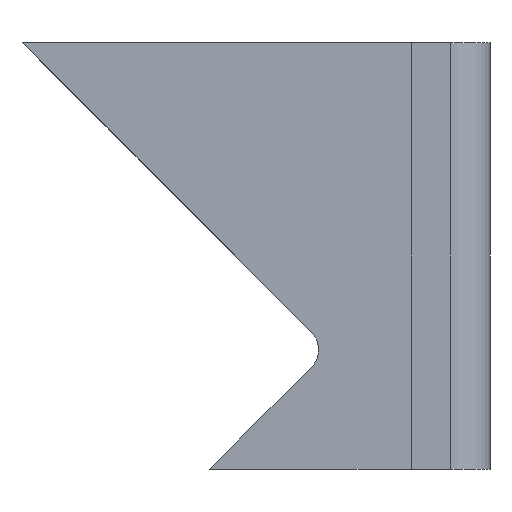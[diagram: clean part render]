
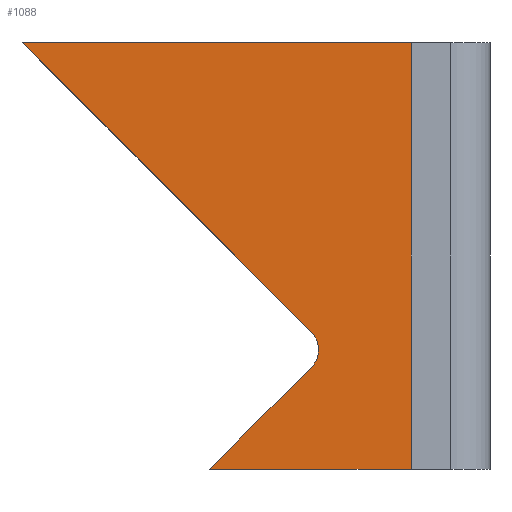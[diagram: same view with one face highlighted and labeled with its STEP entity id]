
A CAD part, front view. The second image highlights one B-rep face of the part: STEP entity #1088.
In plain terms, the highlighted planar face has unit normal (0, -1, 0).
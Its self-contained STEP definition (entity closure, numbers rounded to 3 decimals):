
#139 = VERTEX_POINT('',#140);
#140 = CARTESIAN_POINT('',(4.873,-25.4,-5.818));
#154 = PLANE('',#155);
#155 = AXIS2_PLACEMENT_3D('',#156,#157,#158);
#156 = CARTESIAN_POINT('',(-0.064,-25.4,-5.818));
#157 = DIRECTION('',(0.,0.,1.));
#158 = DIRECTION('',(-1.,0.,0.));
#181 = PLANE('',#182);
#182 = AXIS2_PLACEMENT_3D('',#183,#184,#185);
#183 = CARTESIAN_POINT('',(-5.84,-25.4,5.924));
#184 = DIRECTION('',(0.,-1.,0.));
#185 = DIRECTION('',(0.,0.,-1.));
#345 = CYLINDRICAL_SURFACE('',#346,0.635);
#346 = AXIS2_PLACEMENT_3D('',#347,#348,#349);
#347 = CARTESIAN_POINT('',(1.89,-25.4,-2.788));
#348 = DIRECTION('',(0.,-1.,0.));
#349 = DIRECTION('',(-1.,0.,0.));
#395 = PLANE('',#396);
#396 = AXIS2_PLACEMENT_3D('',#397,#398,#399);
#397 = CARTESIAN_POINT('',(-3.215,-25.4,-8.791));
#398 = DIRECTION('',(0.707,0.,-0.707));
#399 = DIRECTION('',(0.707,0.,0.707));
#445 = PLANE('',#446);
#446 = AXIS2_PLACEMENT_3D('',#447,#448,#449);
#447 = CARTESIAN_POINT('',(-0.064,-25.4,5.));
#448 = DIRECTION('',(0.,0.,-1.));
#449 = DIRECTION('',(1.,0.,0.));
#471 = PLANE('',#472);
#472 = AXIS2_PLACEMENT_3D('',#473,#474,#475);
#473 = CARTESIAN_POINT('',(5.939,-25.4,-5.939));
#474 = DIRECTION('',(-0.707,0.,-0.707));
#475 = DIRECTION('',(0.707,0.,-0.707));
#487 = VERTEX_POINT('',#488);
#488 = CARTESIAN_POINT('',(4.873,-25.4,5.));
#584 = VERTEX_POINT('',#585);
#585 = CARTESIAN_POINT('',(-0.242,-25.4,-5.818));
#606 = EDGE_CURVE('',#584,#139,#607,.T.);
#607 = SURFACE_CURVE('',#608,(#612,#619),.PCURVE_S1.);
#608 = LINE('',#609,#610);
#609 = CARTESIAN_POINT('',(-0.064,-25.4,-5.818));
#610 = VECTOR('',#611,1.);
#611 = DIRECTION('',(1.,0.,0.));
#612 = PCURVE('',#154,#613);
#613 = DEFINITIONAL_REPRESENTATION('',(#614),#618);
#614 = LINE('',#615,#616);
#615 = CARTESIAN_POINT('',(0.,0.));
#616 = VECTOR('',#617,1.);
#617 = DIRECTION('',(-1.,0.));
#618 = ( GEOMETRIC_REPRESENTATION_CONTEXT(2) 
PARAMETRIC_REPRESENTATION_CONTEXT() REPRESENTATION_CONTEXT('2D SPACE',''
  ) );
#619 = PCURVE('',#620,#625);
#620 = PLANE('',#621);
#621 = AXIS2_PLACEMENT_3D('',#622,#623,#624);
#622 = CARTESIAN_POINT('',(-0.064,-25.4,-11.942));
#623 = DIRECTION('',(0.,-1.,0.));
#624 = DIRECTION('',(1.,0.,0.));
#625 = DEFINITIONAL_REPRESENTATION('',(#626),#630);
#626 = LINE('',#627,#628);
#627 = CARTESIAN_POINT('',(0.,6.124));
#628 = VECTOR('',#629,1.);
#629 = DIRECTION('',(1.,0.));
#630 = ( GEOMETRIC_REPRESENTATION_CONTEXT(2) 
PARAMETRIC_REPRESENTATION_CONTEXT() REPRESENTATION_CONTEXT('2D SPACE',''
  ) );
#699 = EDGE_CURVE('',#139,#487,#700,.T.);
#700 = SURFACE_CURVE('',#701,(#705,#712),.PCURVE_S1.);
#701 = LINE('',#702,#703);
#702 = CARTESIAN_POINT('',(4.873,-25.4,-11.942));
#703 = VECTOR('',#704,1.);
#704 = DIRECTION('',(0.,0.,1.));
#705 = PCURVE('',#181,#706);
#706 = DEFINITIONAL_REPRESENTATION('',(#707),#711);
#707 = LINE('',#708,#709);
#708 = CARTESIAN_POINT('',(17.867,10.713));
#709 = VECTOR('',#710,1.);
#710 = DIRECTION('',(-1.,0.));
#711 = ( GEOMETRIC_REPRESENTATION_CONTEXT(2) 
PARAMETRIC_REPRESENTATION_CONTEXT() REPRESENTATION_CONTEXT('2D SPACE',''
  ) );
#712 = PCURVE('',#620,#713);
#713 = DEFINITIONAL_REPRESENTATION('',(#714),#718);
#714 = LINE('',#715,#716);
#715 = CARTESIAN_POINT('',(4.936,0.));
#716 = VECTOR('',#717,1.);
#717 = DIRECTION('',(0.,1.));
#718 = ( GEOMETRIC_REPRESENTATION_CONTEXT(2) 
PARAMETRIC_REPRESENTATION_CONTEXT() REPRESENTATION_CONTEXT('2D SPACE',''
  ) );
#753 = VERTEX_POINT('',#754);
#754 = CARTESIAN_POINT('',(2.339,-25.4,-2.339));
#797 = EDGE_CURVE('',#798,#753,#800,.T.);
#798 = VERTEX_POINT('',#799);
#799 = CARTESIAN_POINT('',(2.339,-25.4,-3.237));
#800 = SURFACE_CURVE('',#801,(#806,#835),.PCURVE_S1.);
#801 = CIRCLE('',#802,0.635);
#802 = AXIS2_PLACEMENT_3D('',#803,#804,#805);
#803 = CARTESIAN_POINT('',(1.89,-25.4,-2.788));
#804 = DIRECTION('',(0.,-1.,0.));
#805 = DIRECTION('',(1.,0.,0.));
#806 = PCURVE('',#345,#807);
#807 = DEFINITIONAL_REPRESENTATION('',(#808),#834);
#808 = B_SPLINE_CURVE_WITH_KNOTS('',3,(#809,#810,#811,#812,#813,#814,
    #815,#816,#817,#818,#819,#820,#821,#822,#823,#824,#825,#826,#827,
    #828,#829,#830,#831,#832,#833),.UNSPECIFIED.,.F.,.F.,(4,1,1,1,1,1,1,
    1,1,1,1,1,1,1,1,1,1,1,1,1,1,1,4),(5.498,5.569,
    5.641,5.712,5.783,5.855,
    5.926,5.998,6.069,6.14,
    6.212,6.283,6.355,6.426,
    6.497,6.569,6.64,6.712,
    6.783,6.854,6.926,6.997,
    7.069),.QUASI_UNIFORM_KNOTS.);
#809 = CARTESIAN_POINT('',(2.356,0.));
#810 = CARTESIAN_POINT('',(2.38,0.));
#811 = CARTESIAN_POINT('',(2.428,0.));
#812 = CARTESIAN_POINT('',(2.499,0.));
#813 = CARTESIAN_POINT('',(2.57,0.));
#814 = CARTESIAN_POINT('',(2.642,0.));
#815 = CARTESIAN_POINT('',(2.713,0.));
#816 = CARTESIAN_POINT('',(2.785,0.));
#817 = CARTESIAN_POINT('',(2.856,0.));
#818 = CARTESIAN_POINT('',(2.927,0.));
#819 = CARTESIAN_POINT('',(2.999,0.));
#820 = CARTESIAN_POINT('',(3.07,0.));
#821 = CARTESIAN_POINT('',(3.142,0.));
#822 = CARTESIAN_POINT('',(3.213,0.));
#823 = CARTESIAN_POINT('',(3.284,0.));
#824 = CARTESIAN_POINT('',(3.356,0.));
#825 = CARTESIAN_POINT('',(3.427,0.));
#826 = CARTESIAN_POINT('',(3.499,0.));
#827 = CARTESIAN_POINT('',(3.57,0.));
#828 = CARTESIAN_POINT('',(3.641,0.));
#829 = CARTESIAN_POINT('',(3.713,0.));
#830 = CARTESIAN_POINT('',(3.784,0.));
#831 = CARTESIAN_POINT('',(3.856,0.));
#832 = CARTESIAN_POINT('',(3.903,0.));
#833 = CARTESIAN_POINT('',(3.927,0.));
#834 = ( GEOMETRIC_REPRESENTATION_CONTEXT(2) 
PARAMETRIC_REPRESENTATION_CONTEXT() REPRESENTATION_CONTEXT('2D SPACE',''
  ) );
#835 = PCURVE('',#620,#836);
#836 = DEFINITIONAL_REPRESENTATION('',(#837),#841);
#837 = CIRCLE('',#838,0.635);
#838 = AXIS2_PLACEMENT_2D('',#839,#840);
#839 = CARTESIAN_POINT('',(1.954,9.154));
#840 = DIRECTION('',(1.,0.));
#841 = ( GEOMETRIC_REPRESENTATION_CONTEXT(2) 
PARAMETRIC_REPRESENTATION_CONTEXT() REPRESENTATION_CONTEXT('2D SPACE',''
  ) );
#892 = EDGE_CURVE('',#798,#584,#893,.T.);
#893 = SURFACE_CURVE('',#894,(#898,#905),.PCURVE_S1.);
#894 = LINE('',#895,#896);
#895 = CARTESIAN_POINT('',(-3.215,-25.4,-8.791));
#896 = VECTOR('',#897,1.);
#897 = DIRECTION('',(-0.707,0.,-0.707));
#898 = PCURVE('',#395,#899);
#899 = DEFINITIONAL_REPRESENTATION('',(#900),#904);
#900 = LINE('',#901,#902);
#901 = CARTESIAN_POINT('',(0.,0.));
#902 = VECTOR('',#903,1.);
#903 = DIRECTION('',(-1.,0.));
#904 = ( GEOMETRIC_REPRESENTATION_CONTEXT(2) 
PARAMETRIC_REPRESENTATION_CONTEXT() REPRESENTATION_CONTEXT('2D SPACE',''
  ) );
#905 = PCURVE('',#620,#906);
#906 = DEFINITIONAL_REPRESENTATION('',(#907),#911);
#907 = LINE('',#908,#909);
#908 = CARTESIAN_POINT('',(-3.151,3.151));
#909 = VECTOR('',#910,1.);
#910 = DIRECTION('',(-0.707,-0.707));
#911 = ( GEOMETRIC_REPRESENTATION_CONTEXT(2) 
PARAMETRIC_REPRESENTATION_CONTEXT() REPRESENTATION_CONTEXT('2D SPACE',''
  ) );
#919 = EDGE_CURVE('',#753,#920,#922,.T.);
#920 = VERTEX_POINT('',#921);
#921 = CARTESIAN_POINT('',(-5.,-25.4,5.));
#922 = SURFACE_CURVE('',#923,(#927,#934),.PCURVE_S1.);
#923 = LINE('',#924,#925);
#924 = CARTESIAN_POINT('',(5.939,-25.4,-5.939));
#925 = VECTOR('',#926,1.);
#926 = DIRECTION('',(-0.707,0.,0.707));
#927 = PCURVE('',#471,#928);
#928 = DEFINITIONAL_REPRESENTATION('',(#929),#933);
#929 = LINE('',#930,#931);
#930 = CARTESIAN_POINT('',(0.,0.));
#931 = VECTOR('',#932,1.);
#932 = DIRECTION('',(-1.,0.));
#933 = ( GEOMETRIC_REPRESENTATION_CONTEXT(2) 
PARAMETRIC_REPRESENTATION_CONTEXT() REPRESENTATION_CONTEXT('2D SPACE',''
  ) );
#934 = PCURVE('',#620,#935);
#935 = DEFINITIONAL_REPRESENTATION('',(#936),#940);
#936 = LINE('',#937,#938);
#937 = CARTESIAN_POINT('',(6.003,6.003));
#938 = VECTOR('',#939,1.);
#939 = DIRECTION('',(-0.707,0.707));
#940 = ( GEOMETRIC_REPRESENTATION_CONTEXT(2) 
PARAMETRIC_REPRESENTATION_CONTEXT() REPRESENTATION_CONTEXT('2D SPACE',''
  ) );
#1067 = EDGE_CURVE('',#487,#920,#1068,.T.);
#1068 = SURFACE_CURVE('',#1069,(#1073,#1080),.PCURVE_S1.);
#1069 = LINE('',#1070,#1071);
#1070 = CARTESIAN_POINT('',(-0.064,-25.4,5.));
#1071 = VECTOR('',#1072,1.);
#1072 = DIRECTION('',(-1.,0.,0.));
#1073 = PCURVE('',#445,#1074);
#1074 = DEFINITIONAL_REPRESENTATION('',(#1075),#1079);
#1075 = LINE('',#1076,#1077);
#1076 = CARTESIAN_POINT('',(0.,0.));
#1077 = VECTOR('',#1078,1.);
#1078 = DIRECTION('',(-1.,0.));
#1079 = ( GEOMETRIC_REPRESENTATION_CONTEXT(2) 
PARAMETRIC_REPRESENTATION_CONTEXT() REPRESENTATION_CONTEXT('2D SPACE',''
  ) );
#1080 = PCURVE('',#620,#1081);
#1081 = DEFINITIONAL_REPRESENTATION('',(#1082),#1086);
#1082 = LINE('',#1083,#1084);
#1083 = CARTESIAN_POINT('',(0.,16.942));
#1084 = VECTOR('',#1085,1.);
#1085 = DIRECTION('',(-1.,0.));
#1086 = ( GEOMETRIC_REPRESENTATION_CONTEXT(2) 
PARAMETRIC_REPRESENTATION_CONTEXT() REPRESENTATION_CONTEXT('2D SPACE',''
  ) );
#1088 = ADVANCED_FACE('',(#1089),#620,.T.);
#1089 = FACE_BOUND('',#1090,.T.);
#1090 = EDGE_LOOP('',(#1091,#1092,#1093,#1094,#1095,#1096));
#1091 = ORIENTED_EDGE('',*,*,#797,.F.);
#1092 = ORIENTED_EDGE('',*,*,#892,.T.);
#1093 = ORIENTED_EDGE('',*,*,#606,.T.);
#1094 = ORIENTED_EDGE('',*,*,#699,.T.);
#1095 = ORIENTED_EDGE('',*,*,#1067,.T.);
#1096 = ORIENTED_EDGE('',*,*,#919,.F.);
